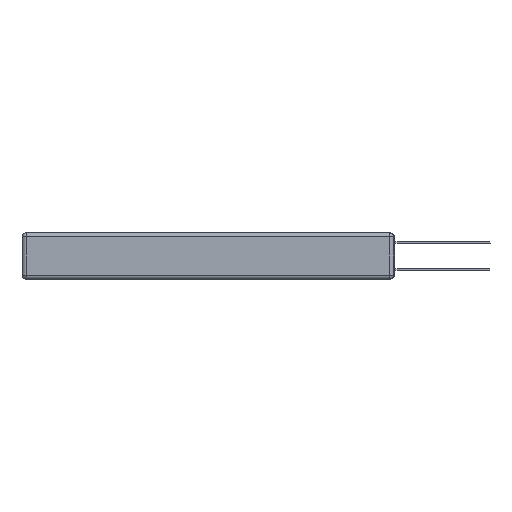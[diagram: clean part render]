
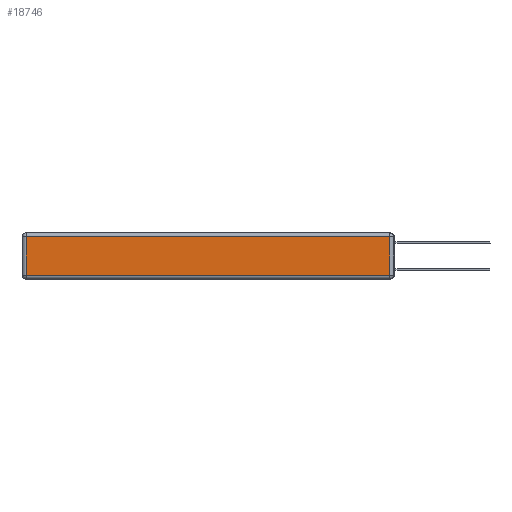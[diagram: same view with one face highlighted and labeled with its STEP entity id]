
A CAD part, left-side view. The second image highlights one B-rep face of the part: STEP entity #18746.
In plain terms, the highlighted planar face has unit normal (-1, 0, 0).
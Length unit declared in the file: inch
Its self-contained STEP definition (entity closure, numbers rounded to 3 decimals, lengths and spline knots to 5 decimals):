
#122 = DIRECTION ( 'NONE',  ( 0., 0., -1. ) ) ;
#417 = EDGE_CURVE ( 'NONE', #18864, #13730, #16023, .T. ) ;
#1281 = LINE ( 'NONE', #11904, #10808 ) ;
#1722 = PLANE ( 'NONE',  #10982 ) ;
#3785 = DIRECTION ( 'NONE',  ( 0., 1., 0. ) ) ;
#4096 = CARTESIAN_POINT ( 'NONE',  ( 0., 0.03, -0.343 ) ) ;
#4658 = ORIENTED_EDGE ( 'NONE', *, *, #12832, .T. ) ;
#5269 = EDGE_CURVE ( 'NONE', #15361, #20411, #18579, .T. ) ;
#5973 = DIRECTION ( 'NONE',  ( 0., 0., 1. ) ) ;
#6577 = CARTESIAN_POINT ( 'NONE',  ( 0., 2.72, -0.03 ) ) ;
#6816 = CARTESIAN_POINT ( 'NONE',  ( 0., 0., -0.343 ) ) ;
#7131 = LINE ( 'NONE', #4096, #14967 ) ;
#8842 = ORIENTED_EDGE ( 'NONE', *, *, #417, .T. ) ;
#10082 = FACE_OUTER_BOUND ( 'NONE', #13990, .T. ) ;
#10808 = VECTOR ( 'NONE', #122, 39.37008 ) ;
#10982 = AXIS2_PLACEMENT_3D ( 'NONE', #6816, #12520, #19408 ) ;
#11238 = VECTOR ( 'NONE', #3785, 39.37008 ) ;
#11904 = CARTESIAN_POINT ( 'NONE',  ( 0., 2.72, -0.343 ) ) ;
#12520 = DIRECTION ( 'NONE',  ( -1., 0., 0. ) ) ;
#12809 = ORIENTED_EDGE ( 'NONE', *, *, #14524, .T. ) ;
#12832 = EDGE_CURVE ( 'NONE', #13730, #15361, #1281, .T. ) ;
#13666 = DIRECTION ( 'NONE',  ( 0., -1., 0. ) ) ;
#13730 = VERTEX_POINT ( 'NONE', #6577 ) ;
#13990 = EDGE_LOOP ( 'NONE', ( #19735, #12809, #8842, #4658 ) ) ;
#14524 = EDGE_CURVE ( 'NONE', #20411, #18864, #7131, .T. ) ;
#14967 = VECTOR ( 'NONE', #5973, 39.37008 ) ;
#15240 = CARTESIAN_POINT ( 'NONE',  ( 0., 2.75, -0.03 ) ) ;
#15361 = VERTEX_POINT ( 'NONE', #18527 ) ;
#16023 = LINE ( 'NONE', #15240, #11238 ) ;
#16837 = CARTESIAN_POINT ( 'NONE',  ( 0., 0.03, -0.313 ) ) ;
#17801 = CARTESIAN_POINT ( 'NONE',  ( 0., 0.03, -0.03 ) ) ;
#18527 = CARTESIAN_POINT ( 'NONE',  ( 0., 2.72, -0.313 ) ) ;
#18579 = LINE ( 'NONE', #22517, #19752 ) ;
#18746 = ADVANCED_FACE ( 'NONE', ( #10082 ), #1722, .T. ) ;
#18864 = VERTEX_POINT ( 'NONE', #17801 ) ;
#19408 = DIRECTION ( 'NONE',  ( 0., 0., 1. ) ) ;
#19735 = ORIENTED_EDGE ( 'NONE', *, *, #5269, .T. ) ;
#19752 = VECTOR ( 'NONE', #13666, 39.37008 ) ;
#20411 = VERTEX_POINT ( 'NONE', #16837 ) ;
#22517 = CARTESIAN_POINT ( 'NONE',  ( 0., 0., -0.313 ) ) ;
